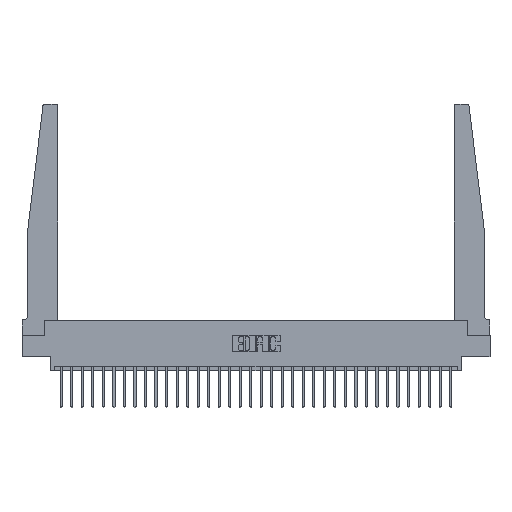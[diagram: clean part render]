
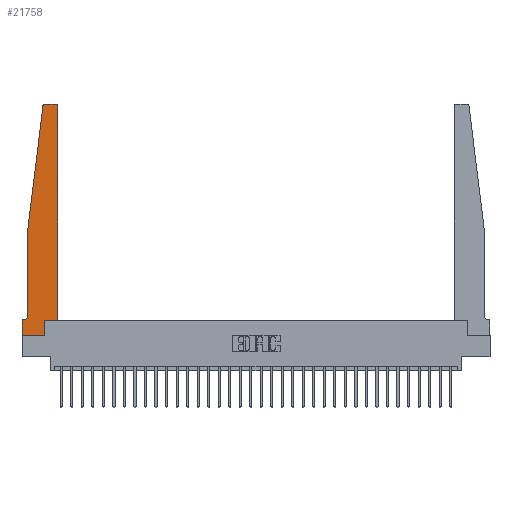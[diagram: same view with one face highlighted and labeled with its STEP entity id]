
A CAD part, top view. The second image highlights one B-rep face of the part: STEP entity #21758.
In plain terms, the highlighted planar face has unit normal (0, 0, 1).
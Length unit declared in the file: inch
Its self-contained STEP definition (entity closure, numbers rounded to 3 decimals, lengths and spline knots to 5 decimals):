
#5 = LINE ( 'NONE', #20944, #23477 ) ;
#948 = VECTOR ( 'NONE', #29805, 39.37008 ) ;
#1078 = ORIENTED_EDGE ( 'NONE', *, *, #28060, .T. ) ;
#1414 = DIRECTION ( 'NONE',  ( 1., 0., 0. ) ) ;
#1537 = VECTOR ( 'NONE', #7550, 39.37008 ) ;
#2124 = LINE ( 'NONE', #23707, #26303 ) ;
#2169 = DIRECTION ( 'NONE',  ( -1., 0., 0. ) ) ;
#2532 = VECTOR ( 'NONE', #4100, 39.37008 ) ;
#2836 = CARTESIAN_POINT ( 'NONE',  ( 0.065, 0.2375, 0.37 ) ) ;
#2872 = CARTESIAN_POINT ( 'NONE',  ( 0.395, 2.72, 0.37 ) ) ;
#3521 = ORIENTED_EDGE ( 'NONE', *, *, #21639, .T. ) ;
#3798 = LINE ( 'NONE', #27892, #27889 ) ;
#3842 = LINE ( 'NONE', #18188, #27229 ) ;
#4100 = DIRECTION ( 'NONE',  ( -1., 0., 0. ) ) ;
#4404 = ORIENTED_EDGE ( 'NONE', *, *, #22249, .T. ) ;
#4717 = EDGE_CURVE ( 'NONE', #9395, #9052, #19003, .T. ) ;
#5119 = CIRCLE ( 'NONE', #21600, 0.03 ) ;
#5230 = DIRECTION ( 'NONE',  ( 1., 0., 0. ) ) ;
#5633 = VERTEX_POINT ( 'NONE', #12340 ) ;
#5754 = CARTESIAN_POINT ( 'NONE',  ( 0.015, 0.2375, 0.37 ) ) ;
#6195 = VERTEX_POINT ( 'NONE', #25513 ) ;
#6778 = CARTESIAN_POINT ( 'NONE',  ( 0.425, 2.72, 0.37 ) ) ;
#7550 = DIRECTION ( 'NONE',  ( 0., -1., 0. ) ) ;
#8076 = AXIS2_PLACEMENT_3D ( 'NONE', #29417, #15508, #1414 ) ;
#8122 = DIRECTION ( 'NONE',  ( -1., 0., 0. ) ) ;
#8540 = EDGE_CURVE ( 'NONE', #12365, #9395, #5, .T. ) ;
#8565 = LINE ( 'NONE', #23893, #1537 ) ;
#8779 = DIRECTION ( 'NONE',  ( 0., 0., 1. ) ) ;
#9052 = VERTEX_POINT ( 'NONE', #23144 ) ;
#9338 = DIRECTION ( 'NONE',  ( 1., 0., 0. ) ) ;
#9395 = VERTEX_POINT ( 'NONE', #24259 ) ;
#9655 = EDGE_CURVE ( 'NONE', #14645, #6195, #15053, .T. ) ;
#9743 = DIRECTION ( 'NONE',  ( -0.122, -0.992, 0. ) ) ;
#9757 = VECTOR ( 'NONE', #11380, 39.37008 ) ;
#9858 = VERTEX_POINT ( 'NONE', #25840 ) ;
#11079 = CARTESIAN_POINT ( 'NONE',  ( 0.395, 2.75, 0.37 ) ) ;
#11335 = ORIENTED_EDGE ( 'NONE', *, *, #8540, .T. ) ;
#11380 = DIRECTION ( 'NONE',  ( 0., 1., 0. ) ) ;
#11388 = VERTEX_POINT ( 'NONE', #14272 ) ;
#11697 = EDGE_CURVE ( 'NONE', #5633, #22557, #26593, .T. ) ;
#12340 = CARTESIAN_POINT ( 'NONE',  ( 0., 0., 0.37 ) ) ;
#12365 = VERTEX_POINT ( 'NONE', #11079 ) ;
#13039 = EDGE_CURVE ( 'NONE', #22557, #9858, #3842, .T. ) ;
#13967 = DIRECTION ( 'NONE',  ( 0., -1., 0. ) ) ;
#14047 = EDGE_CURVE ( 'NONE', #6195, #5633, #8565, .T. ) ;
#14272 = CARTESIAN_POINT ( 'NONE',  ( 0.065, 1.25, 0.37 ) ) ;
#14342 = CIRCLE ( 'NONE', #16509, 0.05 ) ;
#14645 = VERTEX_POINT ( 'NONE', #26201 ) ;
#15053 = LINE ( 'NONE', #18266, #2532 ) ;
#15164 = ORIENTED_EDGE ( 'NONE', *, *, #4717, .T. ) ;
#15270 = VECTOR ( 'NONE', #9338, 39.37008 ) ;
#15508 = DIRECTION ( 'NONE',  ( 0., 0., 1. ) ) ;
#15607 = CARTESIAN_POINT ( 'NONE',  ( 0.2605, 0., 0.37 ) ) ;
#15990 = LINE ( 'NONE', #27546, #9757 ) ;
#16022 = EDGE_CURVE ( 'NONE', #25739, #20148, #15990, .T. ) ;
#16509 = AXIS2_PLACEMENT_3D ( 'NONE', #5754, #22116, #8122 ) ;
#16734 = ORIENTED_EDGE ( 'NONE', *, *, #13039, .T. ) ;
#17112 = ORIENTED_EDGE ( 'NONE', *, *, #16022, .T. ) ;
#17340 = ORIENTED_EDGE ( 'NONE', *, *, #11697, .T. ) ;
#18188 = CARTESIAN_POINT ( 'NONE',  ( 0.2605, 0.18, 0.37 ) ) ;
#18266 = CARTESIAN_POINT ( 'NONE',  ( 0.065, 0.1875, 0.37 ) ) ;
#19003 = CIRCLE ( 'NONE', #24242, 0.03 ) ;
#19281 = DIRECTION ( 'NONE',  ( 0., 0., 1. ) ) ;
#20148 = VERTEX_POINT ( 'NONE', #6778 ) ;
#20248 = ORIENTED_EDGE ( 'NONE', *, *, #14047, .T. ) ;
#20412 = DIRECTION ( 'NONE',  ( 0., 1., 0. ) ) ;
#20944 = CARTESIAN_POINT ( 'NONE',  ( 0.25, 2.75, 0.37 ) ) ;
#21296 = ORIENTED_EDGE ( 'NONE', *, *, #9655, .T. ) ;
#21465 = LINE ( 'NONE', #27956, #15270 ) ;
#21600 = AXIS2_PLACEMENT_3D ( 'NONE', #2872, #19281, #5230 ) ;
#21639 = EDGE_CURVE ( 'NONE', #24805, #14645, #14342, .T. ) ;
#21758 = ADVANCED_FACE ( 'NONE', ( #23078 ), #22423, .T. ) ;
#22116 = DIRECTION ( 'NONE',  ( 0., 0., -1. ) ) ;
#22249 = EDGE_CURVE ( 'NONE', #20148, #12365, #5119, .T. ) ;
#22423 = PLANE ( 'NONE',  #8076 ) ;
#22557 = VERTEX_POINT ( 'NONE', #15607 ) ;
#22754 = CARTESIAN_POINT ( 'NONE',  ( 0.27653, 2.72, 0.37 ) ) ;
#22787 = EDGE_CURVE ( 'NONE', #9052, #11388, #2124, .T. ) ;
#22862 = CARTESIAN_POINT ( 'NONE',  ( 0.425, 0.18, 0.37 ) ) ;
#23078 = FACE_OUTER_BOUND ( 'NONE', #25032, .T. ) ;
#23144 = CARTESIAN_POINT ( 'NONE',  ( 0.24675, 2.72367, 0.37 ) ) ;
#23477 = VECTOR ( 'NONE', #2169, 39.37008 ) ;
#23707 = CARTESIAN_POINT ( 'NONE',  ( 0.065, 1.25, 0.37 ) ) ;
#23893 = CARTESIAN_POINT ( 'NONE',  ( 0., 0., 0.37 ) ) ;
#24242 = AXIS2_PLACEMENT_3D ( 'NONE', #22754, #8779, #25084 ) ;
#24259 = CARTESIAN_POINT ( 'NONE',  ( 0.27653, 2.75, 0.37 ) ) ;
#24653 = EDGE_CURVE ( 'NONE', #9858, #25739, #21465, .T. ) ;
#24805 = VERTEX_POINT ( 'NONE', #2836 ) ;
#25032 = EDGE_LOOP ( 'NONE', ( #11335, #15164, #28509, #1078, #3521, #21296, #20248, #17340, #16734, #29096, #17112, #4404 ) ) ;
#25084 = DIRECTION ( 'NONE',  ( 1., 0., 0. ) ) ;
#25513 = CARTESIAN_POINT ( 'NONE',  ( 0., 0.1875, 0.37 ) ) ;
#25739 = VERTEX_POINT ( 'NONE', #22862 ) ;
#25840 = CARTESIAN_POINT ( 'NONE',  ( 0.2605, 0.18, 0.37 ) ) ;
#26201 = CARTESIAN_POINT ( 'NONE',  ( 0.015, 0.1875, 0.37 ) ) ;
#26303 = VECTOR ( 'NONE', #9743, 39.37008 ) ;
#26593 = LINE ( 'NONE', #27481, #948 ) ;
#27229 = VECTOR ( 'NONE', #20412, 39.37008 ) ;
#27481 = CARTESIAN_POINT ( 'NONE',  ( 0., 0., 0.37 ) ) ;
#27546 = CARTESIAN_POINT ( 'NONE',  ( 0.425, 0.18, 0.37 ) ) ;
#27889 = VECTOR ( 'NONE', #13967, 39.37008 ) ;
#27892 = CARTESIAN_POINT ( 'NONE',  ( 0.065, 1.25, 0.37 ) ) ;
#27956 = CARTESIAN_POINT ( 'NONE',  ( 0.425, 0.18, 0.37 ) ) ;
#28060 = EDGE_CURVE ( 'NONE', #11388, #24805, #3798, .T. ) ;
#28509 = ORIENTED_EDGE ( 'NONE', *, *, #22787, .T. ) ;
#29096 = ORIENTED_EDGE ( 'NONE', *, *, #24653, .T. ) ;
#29417 = CARTESIAN_POINT ( 'NONE',  ( 0., 0.1875, 0.37 ) ) ;
#29805 = DIRECTION ( 'NONE',  ( 1., 0., 0. ) ) ;
